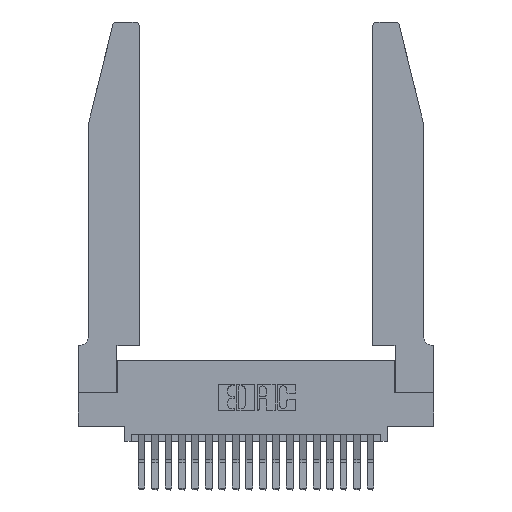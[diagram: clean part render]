
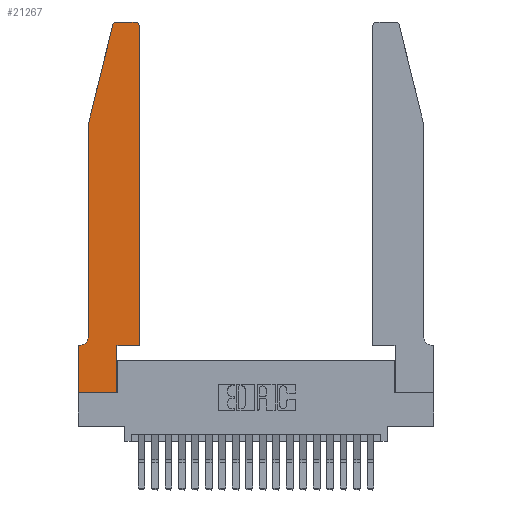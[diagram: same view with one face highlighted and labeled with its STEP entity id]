
A CAD part, top view. The second image highlights one B-rep face of the part: STEP entity #21267.
In plain terms, the highlighted planar face has unit normal (0, 0, 1).
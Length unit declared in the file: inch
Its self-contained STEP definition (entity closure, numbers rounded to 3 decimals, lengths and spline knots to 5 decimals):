
#19 = DIRECTION ( 'NONE',  ( 0., 1., 0. ) ) ;
#123 = EDGE_CURVE ( 'NONE', #17883, #3891, #13750, .T. ) ;
#455 = VERTEX_POINT ( 'NONE', #853 ) ;
#605 = VERTEX_POINT ( 'NONE', #2835 ) ;
#609 = LINE ( 'NONE', #19790, #5422 ) ;
#853 = CARTESIAN_POINT ( 'NONE',  ( 0.0055, 0.35, 0.37 ) ) ;
#1456 = DIRECTION ( 'NONE',  ( 0., 0., 1. ) ) ;
#1676 = ORIENTED_EDGE ( 'NONE', *, *, #12493, .T. ) ;
#2005 = VECTOR ( 'NONE', #7191, 39.37008 ) ;
#2400 = CARTESIAN_POINT ( 'NONE',  ( 0.0755, 2., 0.37 ) ) ;
#2460 = LINE ( 'NONE', #10246, #15601 ) ;
#2689 = ORIENTED_EDGE ( 'NONE', *, *, #9471, .T. ) ;
#2785 = AXIS2_PLACEMENT_3D ( 'NONE', #5483, #17372, #7197 ) ;
#2795 = ORIENTED_EDGE ( 'NONE', *, *, #12445, .T. ) ;
#2835 = CARTESIAN_POINT ( 'NONE',  ( 0.2865, 0., 0.37 ) ) ;
#3319 = DIRECTION ( 'NONE',  ( -0.239, -0.971, 0. ) ) ;
#3353 = ORIENTED_EDGE ( 'NONE', *, *, #22122, .T. ) ;
#3371 = ORIENTED_EDGE ( 'NONE', *, *, #19358, .T. ) ;
#3503 = VERTEX_POINT ( 'NONE', #3621 ) ;
#3621 = CARTESIAN_POINT ( 'NONE',  ( 0.4205, 2.75, 0.37 ) ) ;
#3891 = VERTEX_POINT ( 'NONE', #10023 ) ;
#4106 = ORIENTED_EDGE ( 'NONE', *, *, #6583, .T. ) ;
#4329 = ORIENTED_EDGE ( 'NONE', *, *, #16007, .T. ) ;
#4705 = VECTOR ( 'NONE', #16989, 39.37008 ) ;
#5008 = CARTESIAN_POINT ( 'NONE',  ( 0., 0.35, 0.37 ) ) ;
#5239 = CARTESIAN_POINT ( 'NONE',  ( 0.284, 2.75, 0.37 ) ) ;
#5295 = ORIENTED_EDGE ( 'NONE', *, *, #14855, .T. ) ;
#5422 = VECTOR ( 'NONE', #6201, 39.37008 ) ;
#5483 = CARTESIAN_POINT ( 'NONE',  ( 0.4205, 2.72, 0.37 ) ) ;
#6093 = CIRCLE ( 'NONE', #2785, 0.03 ) ;
#6201 = DIRECTION ( 'NONE',  ( 1., 0., 0. ) ) ;
#6219 = LINE ( 'NONE', #16665, #10726 ) ;
#6504 = DIRECTION ( 'NONE',  ( 0., -1., 0. ) ) ;
#6583 = EDGE_CURVE ( 'NONE', #14411, #12714, #11928, .T. ) ;
#6692 = LINE ( 'NONE', #13922, #2005 ) ;
#7071 = DIRECTION ( 'NONE',  ( 0., 0., -1. ) ) ;
#7146 = CARTESIAN_POINT ( 'NONE',  ( 0.4505, 0.35, 0.37 ) ) ;
#7191 = DIRECTION ( 'NONE',  ( -1., 0., 0. ) ) ;
#7197 = DIRECTION ( 'NONE',  ( 1., 0., 0. ) ) ;
#7406 = CARTESIAN_POINT ( 'NONE',  ( 0.284, 2.72, 0.37 ) ) ;
#7680 = ORIENTED_EDGE ( 'NONE', *, *, #9522, .T. ) ;
#8113 = ORIENTED_EDGE ( 'NONE', *, *, #12130, .T. ) ;
#8463 = CARTESIAN_POINT ( 'NONE',  ( 0.2605, 2.75, 0.37 ) ) ;
#8770 = AXIS2_PLACEMENT_3D ( 'NONE', #17253, #7071, #18966 ) ;
#9471 = EDGE_CURVE ( 'NONE', #3891, #14924, #21716, .T. ) ;
#9522 = EDGE_CURVE ( 'NONE', #14924, #9965, #2460, .T. ) ;
#9598 = FACE_OUTER_BOUND ( 'NONE', #15414, .T. ) ;
#9965 = VERTEX_POINT ( 'NONE', #11635 ) ;
#10023 = CARTESIAN_POINT ( 'NONE',  ( 0.25487, 2.72718, 0.37 ) ) ;
#10246 = CARTESIAN_POINT ( 'NONE',  ( 0.0755, 2., 0.37 ) ) ;
#10281 = CARTESIAN_POINT ( 'NONE',  ( 0.4505, 2.72, 0.37 ) ) ;
#10726 = VECTOR ( 'NONE', #6504, 39.37008 ) ;
#11635 = CARTESIAN_POINT ( 'NONE',  ( 0.0755, 0.42, 0.37 ) ) ;
#11785 = CARTESIAN_POINT ( 'NONE',  ( 0., 0.35, 0.37 ) ) ;
#11842 = PLANE ( 'NONE',  #12133 ) ;
#11879 = CARTESIAN_POINT ( 'NONE',  ( 0.0755, 2., 0.37 ) ) ;
#11928 = LINE ( 'NONE', #13355, #20441 ) ;
#11956 = LINE ( 'NONE', #12553, #20999 ) ;
#12130 = EDGE_CURVE ( 'NONE', #18207, #605, #609, .T. ) ;
#12133 = AXIS2_PLACEMENT_3D ( 'NONE', #5008, #1456, #13524 ) ;
#12445 = EDGE_CURVE ( 'NONE', #9965, #455, #22143, .T. ) ;
#12493 = EDGE_CURVE ( 'NONE', #12714, #19484, #20564, .T. ) ;
#12553 = CARTESIAN_POINT ( 'NONE',  ( 0.2865, 0.35, 0.37 ) ) ;
#12714 = VERTEX_POINT ( 'NONE', #14563 ) ;
#13355 = CARTESIAN_POINT ( 'NONE',  ( 0.4505, 0.35, 0.37 ) ) ;
#13524 = DIRECTION ( 'NONE',  ( 1., 0., 0. ) ) ;
#13683 = EDGE_CURVE ( 'NONE', #455, #17792, #6692, .T. ) ;
#13749 = LINE ( 'NONE', #8463, #4705 ) ;
#13750 = CIRCLE ( 'NONE', #15522, 0.03 ) ;
#13922 = CARTESIAN_POINT ( 'NONE',  ( 0.0755, 0.35, 0.37 ) ) ;
#14199 = CARTESIAN_POINT ( 'NONE',  ( 0.2865, 0.35, 0.37 ) ) ;
#14264 = DIRECTION ( 'NONE',  ( 0., 1., 0. ) ) ;
#14411 = VERTEX_POINT ( 'NONE', #14199 ) ;
#14520 = CARTESIAN_POINT ( 'NONE',  ( 0., 0., 0.37 ) ) ;
#14563 = CARTESIAN_POINT ( 'NONE',  ( 0.4505, 0.35, 0.37 ) ) ;
#14744 = ORIENTED_EDGE ( 'NONE', *, *, #13683, .T. ) ;
#14855 = EDGE_CURVE ( 'NONE', #605, #14411, #11956, .T. ) ;
#14924 = VERTEX_POINT ( 'NONE', #2400 ) ;
#15414 = EDGE_LOOP ( 'NONE', ( #4329, #21644, #2689, #7680, #2795, #14744, #3371, #8113, #5295, #4106, #1676, #3353 ) ) ;
#15522 = AXIS2_PLACEMENT_3D ( 'NONE', #7406, #18511, #21343 ) ;
#15601 = VECTOR ( 'NONE', #18730, 39.37008 ) ;
#16007 = EDGE_CURVE ( 'NONE', #3503, #17883, #13749, .T. ) ;
#16036 = VECTOR ( 'NONE', #19, 39.37008 ) ;
#16665 = CARTESIAN_POINT ( 'NONE',  ( 0., 0., 0.37 ) ) ;
#16989 = DIRECTION ( 'NONE',  ( -1., 0., 0. ) ) ;
#17253 = CARTESIAN_POINT ( 'NONE',  ( 0.0055, 0.42, 0.37 ) ) ;
#17372 = DIRECTION ( 'NONE',  ( 0., 0., 1. ) ) ;
#17792 = VERTEX_POINT ( 'NONE', #11785 ) ;
#17883 = VERTEX_POINT ( 'NONE', #5239 ) ;
#18207 = VERTEX_POINT ( 'NONE', #14520 ) ;
#18511 = DIRECTION ( 'NONE',  ( 0., 0., 1. ) ) ;
#18730 = DIRECTION ( 'NONE',  ( 0., -1., 0. ) ) ;
#18966 = DIRECTION ( 'NONE',  ( -1., 0., 0. ) ) ;
#19358 = EDGE_CURVE ( 'NONE', #17792, #18207, #6219, .T. ) ;
#19484 = VERTEX_POINT ( 'NONE', #10281 ) ;
#19790 = CARTESIAN_POINT ( 'NONE',  ( 0., 0., 0.37 ) ) ;
#20154 = DIRECTION ( 'NONE',  ( 1., 0., 0. ) ) ;
#20441 = VECTOR ( 'NONE', #20154, 39.37008 ) ;
#20564 = LINE ( 'NONE', #7146, #16036 ) ;
#20670 = VECTOR ( 'NONE', #3319, 39.37008 ) ;
#20999 = VECTOR ( 'NONE', #14264, 39.37008 ) ;
#21267 = ADVANCED_FACE ( 'NONE', ( #9598 ), #11842, .T. ) ;
#21343 = DIRECTION ( 'NONE',  ( 1., 0., 0. ) ) ;
#21644 = ORIENTED_EDGE ( 'NONE', *, *, #123, .T. ) ;
#21716 = LINE ( 'NONE', #11879, #20670 ) ;
#22122 = EDGE_CURVE ( 'NONE', #19484, #3503, #6093, .T. ) ;
#22143 = CIRCLE ( 'NONE', #8770, 0.07 ) ;
